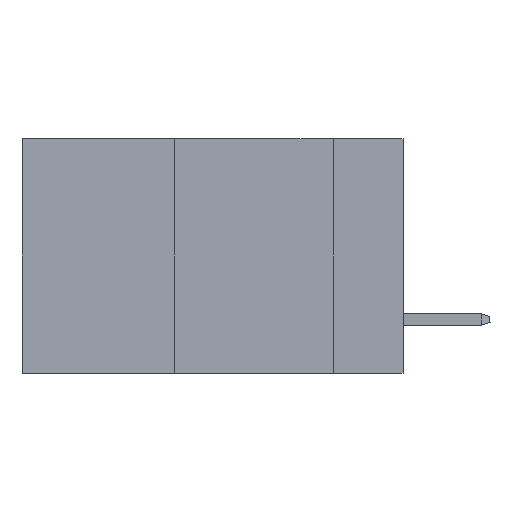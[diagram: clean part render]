
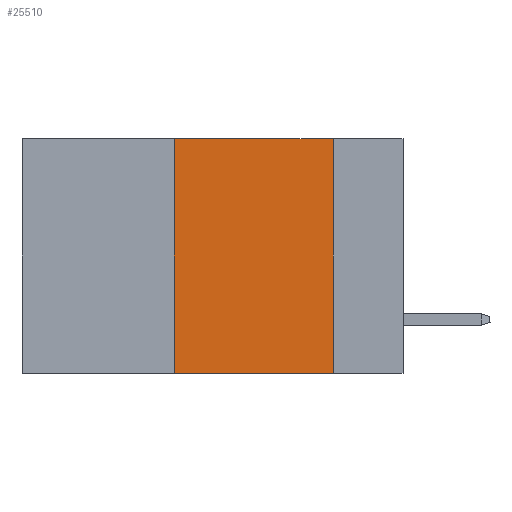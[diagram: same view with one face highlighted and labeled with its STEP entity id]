
A CAD part, left-side view. The second image highlights one B-rep face of the part: STEP entity #25510.
In plain terms, the highlighted planar face has unit normal (-1, 0, 0).
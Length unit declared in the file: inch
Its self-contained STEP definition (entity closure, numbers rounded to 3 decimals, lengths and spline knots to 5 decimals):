
#497 = ORIENTED_EDGE ( 'NONE', *, *, #21201, .F. ) ;
#930 = VERTEX_POINT ( 'NONE', #20885 ) ;
#1867 = VERTEX_POINT ( 'NONE', #5568 ) ;
#1874 = DIRECTION ( 'NONE',  ( 0., -1., 0. ) ) ;
#2357 = LINE ( 'NONE', #18139, #5675 ) ;
#2481 = DIRECTION ( 'NONE',  ( 0., -1., 0. ) ) ;
#2492 = DIRECTION ( 'NONE',  ( 1., 0., 0. ) ) ;
#2826 = EDGE_CURVE ( 'NONE', #11339, #2946, #2357, .T. ) ;
#2946 = VERTEX_POINT ( 'NONE', #5316 ) ;
#4974 = FACE_OUTER_BOUND ( 'NONE', #22486, .T. ) ;
#5109 = VECTOR ( 'NONE', #19109, 39.37008 ) ;
#5316 = CARTESIAN_POINT ( 'NONE',  ( 0., 0.11, -0.37 ) ) ;
#5509 = CARTESIAN_POINT ( 'NONE',  ( 0., 0.36, 0. ) ) ;
#5568 = CARTESIAN_POINT ( 'NONE',  ( 0., 0.36, 0. ) ) ;
#5675 = VECTOR ( 'NONE', #2481, 39.37008 ) ;
#6643 = DIRECTION ( 'NONE',  ( 0., 0., -1. ) ) ;
#7650 = VECTOR ( 'NONE', #1874, 39.37008 ) ;
#7753 = AXIS2_PLACEMENT_3D ( 'NONE', #8839, #2492, #6643 ) ;
#8839 = CARTESIAN_POINT ( 'NONE',  ( 0., 0.6, 0. ) ) ;
#10867 = LINE ( 'NONE', #14698, #5109 ) ;
#11339 = VERTEX_POINT ( 'NONE', #19460 ) ;
#11558 = LINE ( 'NONE', #23911, #7650 ) ;
#12433 = ORIENTED_EDGE ( 'NONE', *, *, #14768, .F. ) ;
#12440 = PLANE ( 'NONE',  #7753 ) ;
#14698 = CARTESIAN_POINT ( 'NONE',  ( 0., 0.11, 0. ) ) ;
#14768 = EDGE_CURVE ( 'NONE', #11339, #1867, #16998, .T. ) ;
#16998 = LINE ( 'NONE', #5509, #18773 ) ;
#18139 = CARTESIAN_POINT ( 'NONE',  ( 0., 0.6, -0.37 ) ) ;
#18773 = VECTOR ( 'NONE', #25325, 39.37008 ) ;
#19109 = DIRECTION ( 'NONE',  ( 0., 0., -1. ) ) ;
#19460 = CARTESIAN_POINT ( 'NONE',  ( 0., 0.36, -0.37 ) ) ;
#20885 = CARTESIAN_POINT ( 'NONE',  ( 0., 0.11, 0. ) ) ;
#21201 = EDGE_CURVE ( 'NONE', #930, #2946, #10867, .T. ) ;
#22401 = EDGE_CURVE ( 'NONE', #1867, #930, #11558, .T. ) ;
#22486 = EDGE_LOOP ( 'NONE', ( #497, #23549, #12433, #25348 ) ) ;
#23549 = ORIENTED_EDGE ( 'NONE', *, *, #22401, .F. ) ;
#23911 = CARTESIAN_POINT ( 'NONE',  ( 0., 0.6, 0. ) ) ;
#25325 = DIRECTION ( 'NONE',  ( 0., 0., 1. ) ) ;
#25348 = ORIENTED_EDGE ( 'NONE', *, *, #2826, .T. ) ;
#25510 = ADVANCED_FACE ( 'NONE', ( #4974 ), #12440, .F. ) ;
